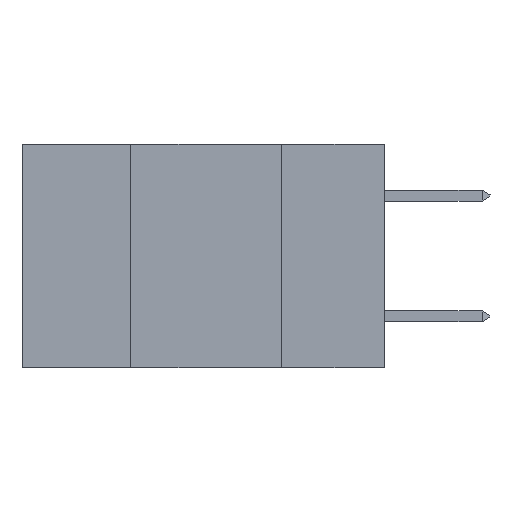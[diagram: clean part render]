
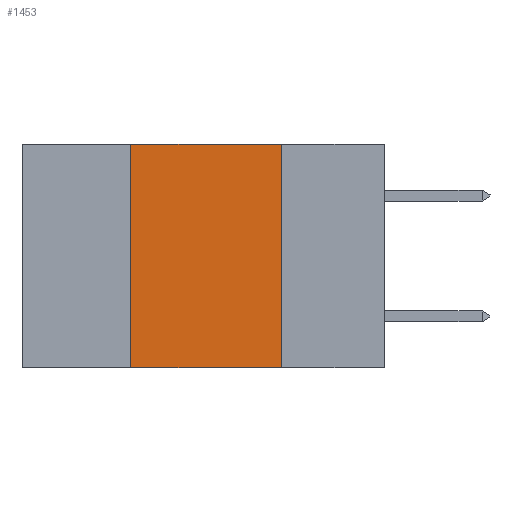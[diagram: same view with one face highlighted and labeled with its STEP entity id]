
A CAD part, left-side view. The second image highlights one B-rep face of the part: STEP entity #1453.
In plain terms, the highlighted planar face has unit normal (-1, 0, 0).
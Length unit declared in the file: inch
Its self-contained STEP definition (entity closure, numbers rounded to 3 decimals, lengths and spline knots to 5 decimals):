
#106 = CARTESIAN_POINT ( 'NONE',  ( 0., 0.42, -0.37 ) ) ;
#342 = EDGE_LOOP ( 'NONE', ( #2812, #427, #5842, #8548 ) ) ;
#427 = ORIENTED_EDGE ( 'NONE', *, *, #7212, .F. ) ;
#824 = CARTESIAN_POINT ( 'NONE',  ( 0., 0.6, -0.37 ) ) ;
#1379 = LINE ( 'NONE', #2344, #9176 ) ;
#1453 = ADVANCED_FACE ( 'NONE', ( #6422 ), #9897, .F. ) ;
#1831 = DIRECTION ( 'NONE',  ( 0., -1., 0. ) ) ;
#1894 = EDGE_CURVE ( 'NONE', #5756, #2030, #12215, .T. ) ;
#2030 = VERTEX_POINT ( 'NONE', #5114 ) ;
#2344 = CARTESIAN_POINT ( 'NONE',  ( 0., 0.17, 0. ) ) ;
#2489 = VERTEX_POINT ( 'NONE', #9402 ) ;
#2812 = ORIENTED_EDGE ( 'NONE', *, *, #5228, .F. ) ;
#3708 = AXIS2_PLACEMENT_3D ( 'NONE', #9928, #9882, #9851 ) ;
#4654 = VERTEX_POINT ( 'NONE', #6557 ) ;
#4707 = VECTOR ( 'NONE', #1831, 39.37008 ) ;
#4922 = VECTOR ( 'NONE', #6624, 39.37008 ) ;
#5114 = CARTESIAN_POINT ( 'NONE',  ( 0., 0.42, 0. ) ) ;
#5228 = EDGE_CURVE ( 'NONE', #2489, #4654, #1379, .T. ) ;
#5564 = EDGE_CURVE ( 'NONE', #5756, #4654, #7436, .T. ) ;
#5756 = VERTEX_POINT ( 'NONE', #106 ) ;
#5842 = ORIENTED_EDGE ( 'NONE', *, *, #1894, .F. ) ;
#6340 = CARTESIAN_POINT ( 'NONE',  ( 0., 0.42, 0. ) ) ;
#6419 = DIRECTION ( 'NONE',  ( 0., 0., 1. ) ) ;
#6422 = FACE_OUTER_BOUND ( 'NONE', #342, .T. ) ;
#6557 = CARTESIAN_POINT ( 'NONE',  ( 0., 0.17, -0.37 ) ) ;
#6624 = DIRECTION ( 'NONE',  ( 0., -1., 0. ) ) ;
#7212 = EDGE_CURVE ( 'NONE', #2030, #2489, #10561, .T. ) ;
#7436 = LINE ( 'NONE', #824, #4707 ) ;
#8440 = DIRECTION ( 'NONE',  ( 0., 0., -1. ) ) ;
#8548 = ORIENTED_EDGE ( 'NONE', *, *, #5564, .T. ) ;
#9176 = VECTOR ( 'NONE', #8440, 39.37008 ) ;
#9402 = CARTESIAN_POINT ( 'NONE',  ( 0., 0.17, 0. ) ) ;
#9851 = DIRECTION ( 'NONE',  ( 0., 0., -1. ) ) ;
#9882 = DIRECTION ( 'NONE',  ( 1., 0., 0. ) ) ;
#9897 = PLANE ( 'NONE',  #3708 ) ;
#9928 = CARTESIAN_POINT ( 'NONE',  ( 0., 0.6, 0. ) ) ;
#10561 = LINE ( 'NONE', #12489, #4922 ) ;
#11921 = VECTOR ( 'NONE', #6419, 39.37008 ) ;
#12215 = LINE ( 'NONE', #6340, #11921 ) ;
#12489 = CARTESIAN_POINT ( 'NONE',  ( 0., 0.6, 0. ) ) ;
